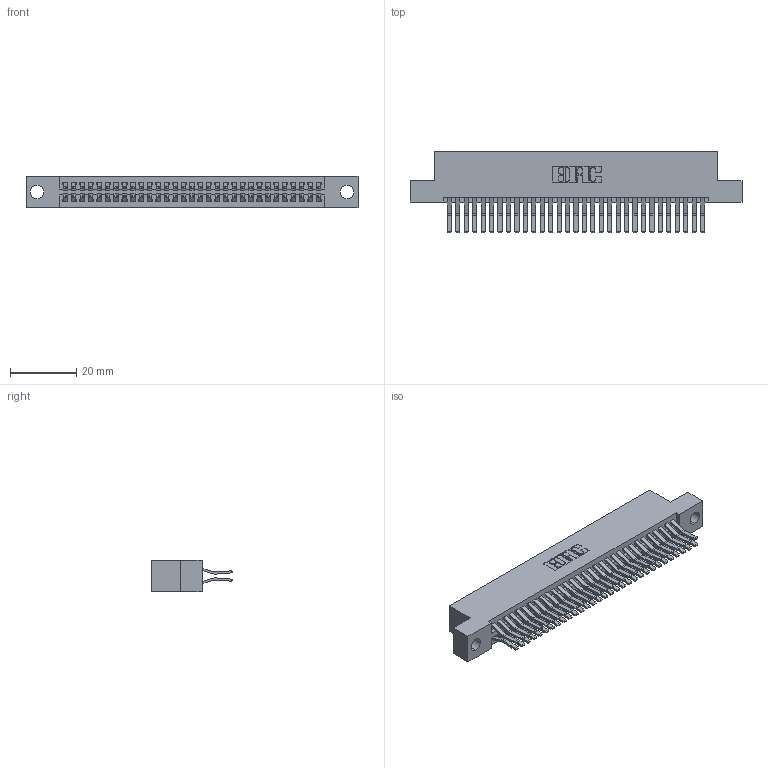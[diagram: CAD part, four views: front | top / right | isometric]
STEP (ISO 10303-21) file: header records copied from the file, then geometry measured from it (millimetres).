
FILE_DESCRIPTION (( 'STEP AP203' ), '1' );
FILE_NAME ('345-062-560-204.STEP', '2018-09-27T23:26:44', ( '' ), ( '' ), 'SwSTEP 2.0', 'SolidWorks 2016', '' );
FILE_SCHEMA (( 'CONFIG_CONTROL_DESIGN' ));
Length unit declared in the file: inch
Products named in the file (3): 345-062-560-204; 345 Part_Flush Mounting Lugs - 0.156 Dia-TH; 345-292-001_560 Tail
Assembly tree (63 placements, depth 2):
  345-062-560-204
    345 Part_Flush Mounting Lugs - 0.156 Dia-TH
    345-292-001_560 Tail  x62
Bounding box: 99.95 x 24.45 x 9.4 mm (x, y, z)
Volume: 9925.6 mm3; surface area: 15319 mm2
Topology: 63 solids, 63 shells, 3350 faces, 9951 edges, 6550 vertices
Faces by surface type: plane 2126, cylinder 1224
Entity records: 25895 total; most frequent: CARTESIAN_POINT 4352, ORIENTED_EDGE 4286, DIRECTION 3855, EDGE_CURVE 2143, LINE 1883, VECTOR 1883, VERTEX_POINT 1426, AXIS2_PLACEMENT_3D 986
